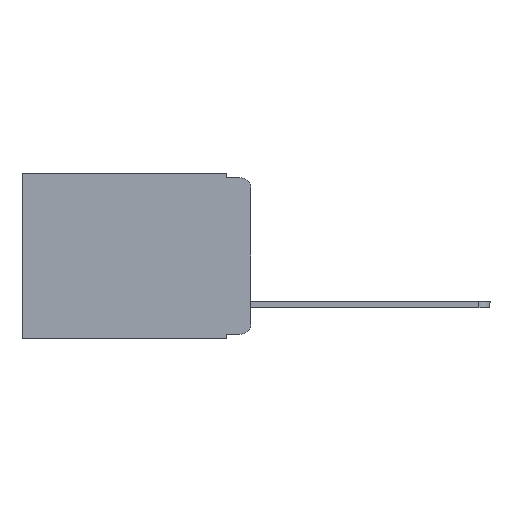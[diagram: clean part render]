
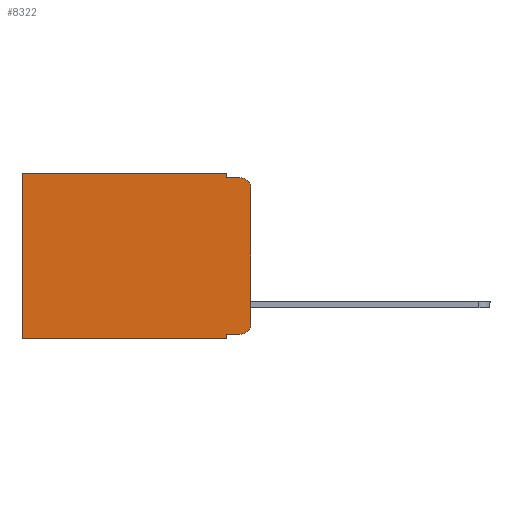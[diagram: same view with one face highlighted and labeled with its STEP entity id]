
A CAD part, left-side view. The second image highlights one B-rep face of the part: STEP entity #8322.
In plain terms, the highlighted planar face has unit normal (-1, 0, 0).
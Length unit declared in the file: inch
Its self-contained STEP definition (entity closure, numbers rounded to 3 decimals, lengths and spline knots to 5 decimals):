
#40 = EDGE_CURVE ( 'NONE', #7102, #20269, #17533, .T. ) ;
#192 = CIRCLE ( 'NONE', #10004, 0.02 ) ;
#579 = VERTEX_POINT ( 'NONE', #6839 ) ;
#620 = CIRCLE ( 'NONE', #12514, 0.02 ) ;
#915 = CARTESIAN_POINT ( 'NONE',  ( 0.298, 0.02, -0.313 ) ) ;
#916 = ORIENTED_EDGE ( 'NONE', *, *, #7120, .F. ) ;
#1537 = DIRECTION ( 'NONE',  ( 0., 0., -1. ) ) ;
#1965 = CARTESIAN_POINT ( 'NONE',  ( 0.298, 0.473, 0. ) ) ;
#2242 = DIRECTION ( 'NONE',  ( 0., -1., 0. ) ) ;
#2436 = ORIENTED_EDGE ( 'NONE', *, *, #16067, .F. ) ;
#2518 = VERTEX_POINT ( 'NONE', #12753 ) ;
#3736 = ORIENTED_EDGE ( 'NONE', *, *, #13836, .T. ) ;
#3833 = CARTESIAN_POINT ( 'NONE',  ( 0.298, 0.051, -0.333 ) ) ;
#3939 = CARTESIAN_POINT ( 'NONE',  ( 0.298, 0.051, -0.01 ) ) ;
#4000 = EDGE_CURVE ( 'NONE', #17686, #20315, #10654, .T. ) ;
#4475 = CARTESIAN_POINT ( 'NONE',  ( 0.298, 0., 0. ) ) ;
#4945 = VECTOR ( 'NONE', #15147, 39.37008 ) ;
#4950 = VECTOR ( 'NONE', #2242, 39.37008 ) ;
#5307 = VECTOR ( 'NONE', #1537, 39.37008 ) ;
#5598 = DIRECTION ( 'NONE',  ( -1., 0., 0. ) ) ;
#6106 = VERTEX_POINT ( 'NONE', #15086 ) ;
#6262 = CARTESIAN_POINT ( 'NONE',  ( 0.298, 0., 0. ) ) ;
#6515 = ORIENTED_EDGE ( 'NONE', *, *, #11647, .F. ) ;
#6582 = DIRECTION ( 'NONE',  ( 0., 0., -1. ) ) ;
#6747 = VERTEX_POINT ( 'NONE', #3833 ) ;
#6839 = CARTESIAN_POINT ( 'NONE',  ( 0.298, 0.473, -0.343 ) ) ;
#7102 = VERTEX_POINT ( 'NONE', #8066 ) ;
#7120 = EDGE_CURVE ( 'NONE', #2518, #579, #19154, .T. ) ;
#7122 = VECTOR ( 'NONE', #14774, 39.37008 ) ;
#7138 = VECTOR ( 'NONE', #6582, 39.37008 ) ;
#7470 = DIRECTION ( 'NONE',  ( 0., 0., -1. ) ) ;
#7585 = EDGE_CURVE ( 'NONE', #7102, #20694, #17908, .T. ) ;
#7792 = EDGE_CURVE ( 'NONE', #20269, #579, #20369, .T. ) ;
#7861 = DIRECTION ( 'NONE',  ( 0., 1., 0. ) ) ;
#7871 = LINE ( 'NONE', #8075, #7122 ) ;
#7999 = CARTESIAN_POINT ( 'NONE',  ( 0.298, 0.051, -0.01 ) ) ;
#8066 = CARTESIAN_POINT ( 'NONE',  ( 0.298, 0.051, 0. ) ) ;
#8075 = CARTESIAN_POINT ( 'NONE',  ( 0.298, 0.051, -0.333 ) ) ;
#8322 = ADVANCED_FACE ( 'NONE', ( #14045 ), #19163, .F. ) ;
#8875 = CARTESIAN_POINT ( 'NONE',  ( 0.298, 0.473, 0. ) ) ;
#9229 = EDGE_CURVE ( 'NONE', #17686, #18758, #192, .T. ) ;
#9771 = LINE ( 'NONE', #11168, #7138 ) ;
#10004 = AXIS2_PLACEMENT_3D ( 'NONE', #12033, #16726, #19921 ) ;
#10654 = LINE ( 'NONE', #18430, #15006 ) ;
#10791 = ORIENTED_EDGE ( 'NONE', *, *, #4000, .F. ) ;
#11168 = CARTESIAN_POINT ( 'NONE',  ( 0.298, 0.051, 0. ) ) ;
#11374 = CARTESIAN_POINT ( 'NONE',  ( 0.298, 0.02, -0.01 ) ) ;
#11647 = EDGE_CURVE ( 'NONE', #20694, #18758, #13728, .T. ) ;
#12033 = CARTESIAN_POINT ( 'NONE',  ( 0.298, 0.02, -0.03 ) ) ;
#12084 = DIRECTION ( 'NONE',  ( 0., 0., -1. ) ) ;
#12453 = DIRECTION ( 'NONE',  ( 0., 0., -1. ) ) ;
#12514 = AXIS2_PLACEMENT_3D ( 'NONE', #915, #5598, #12084 ) ;
#12744 = DIRECTION ( 'NONE',  ( 0., 1., 0. ) ) ;
#12753 = CARTESIAN_POINT ( 'NONE',  ( 0.298, 0.051, -0.343 ) ) ;
#13449 = CARTESIAN_POINT ( 'NONE',  ( 0.298, 0., -0.313 ) ) ;
#13728 = LINE ( 'NONE', #3939, #4950 ) ;
#13836 = EDGE_CURVE ( 'NONE', #6106, #20315, #620, .T. ) ;
#14045 = FACE_OUTER_BOUND ( 'NONE', #16670, .T. ) ;
#14205 = ORIENTED_EDGE ( 'NONE', *, *, #16038, .T. ) ;
#14234 = CARTESIAN_POINT ( 'NONE',  ( 0.298, 0., -0.03 ) ) ;
#14398 = ORIENTED_EDGE ( 'NONE', *, *, #7792, .T. ) ;
#14774 = DIRECTION ( 'NONE',  ( 0., -1., 0. ) ) ;
#15006 = VECTOR ( 'NONE', #7470, 39.37008 ) ;
#15047 = ORIENTED_EDGE ( 'NONE', *, *, #7585, .F. ) ;
#15086 = CARTESIAN_POINT ( 'NONE',  ( 0.298, 0.02, -0.333 ) ) ;
#15147 = DIRECTION ( 'NONE',  ( 0., 0., -1. ) ) ;
#15182 = AXIS2_PLACEMENT_3D ( 'NONE', #4475, #15650, #12453 ) ;
#15208 = CARTESIAN_POINT ( 'NONE',  ( 0.298, 0., -0.343 ) ) ;
#15650 = DIRECTION ( 'NONE',  ( 1., 0., 0. ) ) ;
#16038 = EDGE_CURVE ( 'NONE', #6747, #6106, #7871, .T. ) ;
#16067 = EDGE_CURVE ( 'NONE', #6747, #2518, #9771, .T. ) ;
#16163 = ORIENTED_EDGE ( 'NONE', *, *, #40, .T. ) ;
#16670 = EDGE_LOOP ( 'NONE', ( #10791, #20839, #6515, #15047, #16163, #14398, #916, #2436, #14205, #3736 ) ) ;
#16726 = DIRECTION ( 'NONE',  ( -1., 0., 0. ) ) ;
#17180 = VECTOR ( 'NONE', #12744, 39.37008 ) ;
#17533 = LINE ( 'NONE', #6262, #17180 ) ;
#17686 = VERTEX_POINT ( 'NONE', #14234 ) ;
#17908 = LINE ( 'NONE', #19623, #5307 ) ;
#18430 = CARTESIAN_POINT ( 'NONE',  ( 0.298, 0., 0. ) ) ;
#18758 = VERTEX_POINT ( 'NONE', #11374 ) ;
#19154 = LINE ( 'NONE', #15208, #19851 ) ;
#19163 = PLANE ( 'NONE',  #15182 ) ;
#19623 = CARTESIAN_POINT ( 'NONE',  ( 0.298, 0.051, 0. ) ) ;
#19851 = VECTOR ( 'NONE', #7861, 39.37008 ) ;
#19921 = DIRECTION ( 'NONE',  ( 0., 0., -1. ) ) ;
#20269 = VERTEX_POINT ( 'NONE', #1965 ) ;
#20315 = VERTEX_POINT ( 'NONE', #13449 ) ;
#20369 = LINE ( 'NONE', #8875, #4945 ) ;
#20694 = VERTEX_POINT ( 'NONE', #7999 ) ;
#20839 = ORIENTED_EDGE ( 'NONE', *, *, #9229, .T. ) ;
